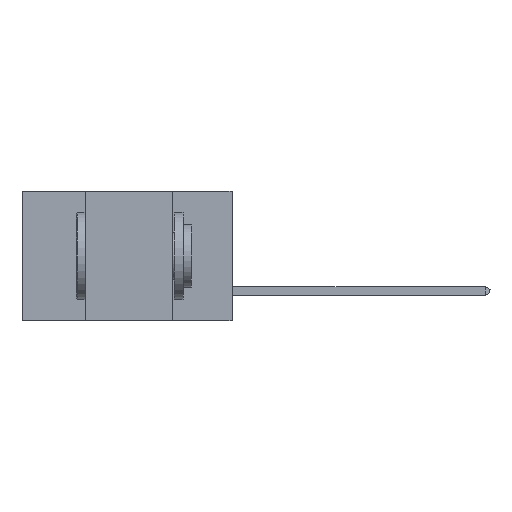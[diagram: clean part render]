
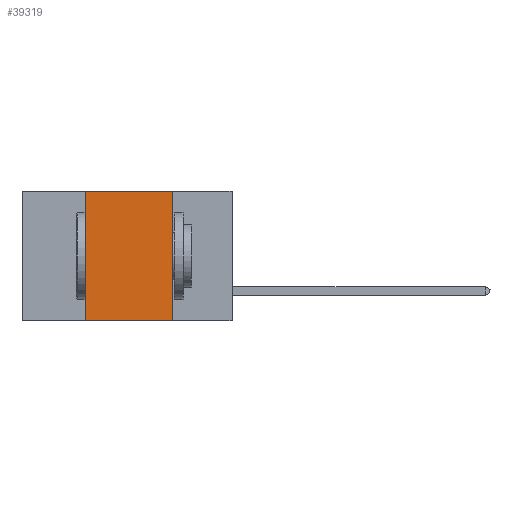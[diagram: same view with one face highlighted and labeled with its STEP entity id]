
A CAD part, left-side view. The second image highlights one B-rep face of the part: STEP entity #39319.
In plain terms, the highlighted planar face has unit normal (-1, 0, 0).
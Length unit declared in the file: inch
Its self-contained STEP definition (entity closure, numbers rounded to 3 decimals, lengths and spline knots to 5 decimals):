
#852 = VERTEX_POINT ( 'NONE', #11893 ) ;
#937 = CARTESIAN_POINT ( 'NONE',  ( 0., 0.17, -0.37 ) ) ;
#4992 = DIRECTION ( 'NONE',  ( 0., -1., 0. ) ) ;
#5202 = VERTEX_POINT ( 'NONE', #27300 ) ;
#8772 = VECTOR ( 'NONE', #4992, 39.37008 ) ;
#9174 = LINE ( 'NONE', #17099, #36965 ) ;
#9206 = CARTESIAN_POINT ( 'NONE',  ( 0., 0.42, 0. ) ) ;
#11448 = FACE_OUTER_BOUND ( 'NONE', #49385, .T. ) ;
#11893 = CARTESIAN_POINT ( 'NONE',  ( 0., 0.42, 0. ) ) ;
#12410 = CARTESIAN_POINT ( 'NONE',  ( 0., 0.6, 0. ) ) ;
#12500 = CARTESIAN_POINT ( 'NONE',  ( 0., 0.6, 0. ) ) ;
#12549 = PLANE ( 'NONE',  #46125 ) ;
#14739 = ORIENTED_EDGE ( 'NONE', *, *, #35041, .F. ) ;
#17099 = CARTESIAN_POINT ( 'NONE',  ( 0., 0.6, -0.37 ) ) ;
#18129 = CARTESIAN_POINT ( 'NONE',  ( 0., 0.17, 0. ) ) ;
#20454 = VECTOR ( 'NONE', #24325, 39.37008 ) ;
#22149 = DIRECTION ( 'NONE',  ( 0., 0., -1. ) ) ;
#23564 = EDGE_CURVE ( 'NONE', #5202, #852, #43187, .T. ) ;
#24325 = DIRECTION ( 'NONE',  ( 0., 0., 1. ) ) ;
#24342 = DIRECTION ( 'NONE',  ( 0., -1., 0. ) ) ;
#24476 = DIRECTION ( 'NONE',  ( 0., 0., -1. ) ) ;
#25048 = EDGE_CURVE ( 'NONE', #38575, #34338, #47904, .T. ) ;
#27300 = CARTESIAN_POINT ( 'NONE',  ( 0., 0.42, -0.37 ) ) ;
#27537 = CARTESIAN_POINT ( 'NONE',  ( 0., 0.17, 0. ) ) ;
#29948 = ORIENTED_EDGE ( 'NONE', *, *, #46234, .T. ) ;
#32486 = ORIENTED_EDGE ( 'NONE', *, *, #23564, .F. ) ;
#34338 = VERTEX_POINT ( 'NONE', #937 ) ;
#35041 = EDGE_CURVE ( 'NONE', #852, #38575, #41875, .T. ) ;
#36965 = VECTOR ( 'NONE', #24342, 39.37008 ) ;
#38575 = VERTEX_POINT ( 'NONE', #27537 ) ;
#39319 = ADVANCED_FACE ( 'NONE', ( #11448 ), #12549, .F. ) ;
#40277 = ORIENTED_EDGE ( 'NONE', *, *, #25048, .F. ) ;
#41875 = LINE ( 'NONE', #12500, #8772 ) ;
#43187 = LINE ( 'NONE', #9206, #20454 ) ;
#46125 = AXIS2_PLACEMENT_3D ( 'NONE', #12410, #47012, #24476 ) ;
#46234 = EDGE_CURVE ( 'NONE', #5202, #34338, #9174, .T. ) ;
#46656 = VECTOR ( 'NONE', #22149, 39.37008 ) ;
#47012 = DIRECTION ( 'NONE',  ( 1., 0., 0. ) ) ;
#47904 = LINE ( 'NONE', #18129, #46656 ) ;
#49385 = EDGE_LOOP ( 'NONE', ( #40277, #14739, #32486, #29948 ) ) ;
